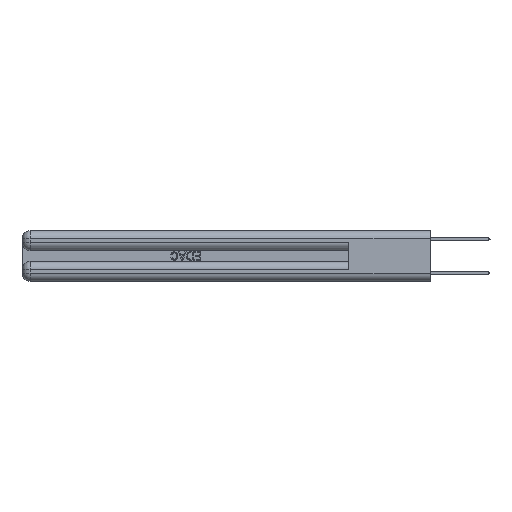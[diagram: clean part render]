
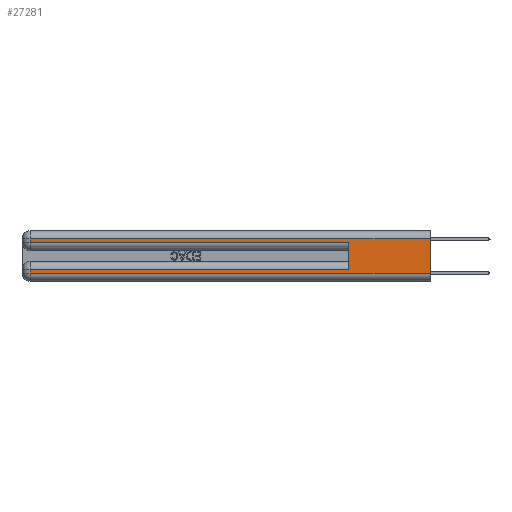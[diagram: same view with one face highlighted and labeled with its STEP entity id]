
A CAD part, left-side view. The second image highlights one B-rep face of the part: STEP entity #27281.
In plain terms, the highlighted planar face has unit normal (-1, 0, 0).
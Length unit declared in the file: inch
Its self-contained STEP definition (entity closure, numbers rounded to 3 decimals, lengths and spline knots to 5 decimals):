
#84 = LINE ( 'NONE', #5059, #22037 ) ;
#183 = LINE ( 'NONE', #3159, #20849 ) ;
#1521 = CARTESIAN_POINT ( 'NONE',  ( 0., 0., 0.37 ) ) ;
#1704 = EDGE_CURVE ( 'NONE', #4344, #32507, #5366, .T. ) ;
#1985 = CARTESIAN_POINT ( 'NONE',  ( 0., 0.6, 0.285 ) ) ;
#2120 = VERTEX_POINT ( 'NONE', #18006 ) ;
#2609 = ORIENTED_EDGE ( 'NONE', *, *, #10044, .T. ) ;
#3159 = CARTESIAN_POINT ( 'NONE',  ( 0., 0.6, 0.145 ) ) ;
#4031 = EDGE_CURVE ( 'NONE', #32225, #26299, #23405, .T. ) ;
#4344 = VERTEX_POINT ( 'NONE', #10515 ) ;
#5059 = CARTESIAN_POINT ( 'NONE',  ( 0., 2.94, 0.37 ) ) ;
#5177 = VECTOR ( 'NONE', #20921, 39.37008 ) ;
#5366 = LINE ( 'NONE', #28243, #11262 ) ;
#5676 = AXIS2_PLACEMENT_3D ( 'NONE', #1521, #9128, #11584 ) ;
#6276 = VECTOR ( 'NONE', #13684, 39.37008 ) ;
#6440 = LINE ( 'NONE', #14347, #6276 ) ;
#7235 = LINE ( 'NONE', #26561, #13905 ) ;
#7337 = EDGE_CURVE ( 'NONE', #13780, #32507, #183, .T. ) ;
#9128 = DIRECTION ( 'NONE',  ( 1., 0., 0. ) ) ;
#9148 = DIRECTION ( 'NONE',  ( 0., 1., 0. ) ) ;
#10044 = EDGE_CURVE ( 'NONE', #18471, #26299, #25314, .T. ) ;
#10515 = CARTESIAN_POINT ( 'NONE',  ( 0., 2.94, 0.285 ) ) ;
#10883 = CARTESIAN_POINT ( 'NONE',  ( 0., 0., 0.37 ) ) ;
#11095 = VECTOR ( 'NONE', #9148, 39.37008 ) ;
#11262 = VECTOR ( 'NONE', #27754, 39.37008 ) ;
#11584 = DIRECTION ( 'NONE',  ( 0., 0., -1. ) ) ;
#12301 = DIRECTION ( 'NONE',  ( 0., 0., -1. ) ) ;
#12524 = EDGE_CURVE ( 'NONE', #13780, #20277, #6440, .T. ) ;
#12586 = ORIENTED_EDGE ( 'NONE', *, *, #28335, .T. ) ;
#13684 = DIRECTION ( 'NONE',  ( 0., 1., 0. ) ) ;
#13780 = VERTEX_POINT ( 'NONE', #15520 ) ;
#13905 = VECTOR ( 'NONE', #22374, 39.37008 ) ;
#14229 = ORIENTED_EDGE ( 'NONE', *, *, #21291, .T. ) ;
#14347 = CARTESIAN_POINT ( 'NONE',  ( 0., 0., 0.085 ) ) ;
#15094 = DIRECTION ( 'NONE',  ( 0., -1., 0. ) ) ;
#15365 = DIRECTION ( 'NONE',  ( 0., 0., 1. ) ) ;
#15406 = EDGE_CURVE ( 'NONE', #32225, #2120, #32004, .T. ) ;
#15520 = CARTESIAN_POINT ( 'NONE',  ( 0., 0.6, 0.085 ) ) ;
#17177 = PLANE ( 'NONE',  #5676 ) ;
#18006 = CARTESIAN_POINT ( 'NONE',  ( 0., 2.94, 0.31 ) ) ;
#18471 = VERTEX_POINT ( 'NONE', #23389 ) ;
#19477 = EDGE_LOOP ( 'NONE', ( #31006, #28183, #12586, #31457, #28043, #30545, #14229, #2609 ) ) ;
#20277 = VERTEX_POINT ( 'NONE', #23843 ) ;
#20849 = VECTOR ( 'NONE', #15365, 39.37008 ) ;
#20921 = DIRECTION ( 'NONE',  ( 0., 0., -1. ) ) ;
#21291 = EDGE_CURVE ( 'NONE', #20277, #18471, #7235, .T. ) ;
#22037 = VECTOR ( 'NONE', #12301, 39.37008 ) ;
#22374 = DIRECTION ( 'NONE',  ( 0., 0., -1. ) ) ;
#23389 = CARTESIAN_POINT ( 'NONE',  ( 0., 2.94, 0.06 ) ) ;
#23405 = LINE ( 'NONE', #10883, #5177 ) ;
#23843 = CARTESIAN_POINT ( 'NONE',  ( 0., 2.94, 0.085 ) ) ;
#24297 = CARTESIAN_POINT ( 'NONE',  ( 0., 0., 0.31 ) ) ;
#25314 = LINE ( 'NONE', #29746, #28250 ) ;
#26299 = VERTEX_POINT ( 'NONE', #28672 ) ;
#26561 = CARTESIAN_POINT ( 'NONE',  ( 0., 2.94, 0.37 ) ) ;
#27281 = ADVANCED_FACE ( 'NONE', ( #31504 ), #17177, .F. ) ;
#27754 = DIRECTION ( 'NONE',  ( 0., -1., 0. ) ) ;
#28043 = ORIENTED_EDGE ( 'NONE', *, *, #7337, .F. ) ;
#28183 = ORIENTED_EDGE ( 'NONE', *, *, #15406, .T. ) ;
#28243 = CARTESIAN_POINT ( 'NONE',  ( 0., 0., 0.285 ) ) ;
#28250 = VECTOR ( 'NONE', #15094, 39.37008 ) ;
#28335 = EDGE_CURVE ( 'NONE', #2120, #4344, #84, .T. ) ;
#28672 = CARTESIAN_POINT ( 'NONE',  ( 0., 0., 0.06 ) ) ;
#29746 = CARTESIAN_POINT ( 'NONE',  ( 0., 0., 0.06 ) ) ;
#30175 = CARTESIAN_POINT ( 'NONE',  ( 0., 0., 0.31 ) ) ;
#30545 = ORIENTED_EDGE ( 'NONE', *, *, #12524, .T. ) ;
#31006 = ORIENTED_EDGE ( 'NONE', *, *, #4031, .F. ) ;
#31457 = ORIENTED_EDGE ( 'NONE', *, *, #1704, .T. ) ;
#31504 = FACE_OUTER_BOUND ( 'NONE', #19477, .T. ) ;
#32004 = LINE ( 'NONE', #24297, #11095 ) ;
#32225 = VERTEX_POINT ( 'NONE', #30175 ) ;
#32507 = VERTEX_POINT ( 'NONE', #1985 ) ;
